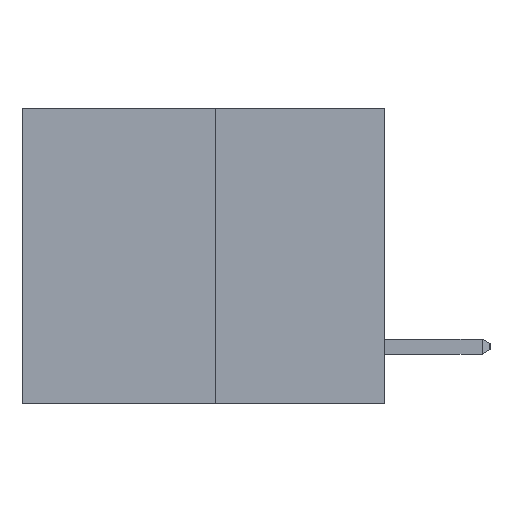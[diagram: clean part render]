
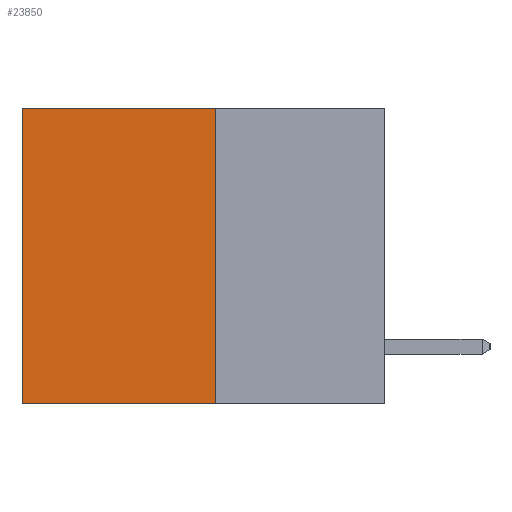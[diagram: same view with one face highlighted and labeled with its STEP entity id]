
A CAD part, left-side view. The second image highlights one B-rep face of the part: STEP entity #23850.
In plain terms, the highlighted planar face has unit normal (-1, 0, 0).
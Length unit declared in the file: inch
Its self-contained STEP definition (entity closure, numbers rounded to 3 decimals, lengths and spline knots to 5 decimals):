
#1382 = FACE_OUTER_BOUND ( 'NONE', #16601, .T. ) ;
#1690 = LINE ( 'NONE', #16212, #13987 ) ;
#6266 = CARTESIAN_POINT ( 'NONE',  ( 0.3165, 0.28, -0.49 ) ) ;
#6625 = VERTEX_POINT ( 'NONE', #8725 ) ;
#7348 = LINE ( 'NONE', #9568, #12808 ) ;
#7828 = PLANE ( 'NONE',  #15350 ) ;
#8725 = CARTESIAN_POINT ( 'NONE',  ( 0.3165, 0.28, 0. ) ) ;
#9127 = VERTEX_POINT ( 'NONE', #21963 ) ;
#9568 = CARTESIAN_POINT ( 'NONE',  ( 0.3165, 0.6, -0.49 ) ) ;
#9924 = DIRECTION ( 'NONE',  ( 0., 0., -1. ) ) ;
#10019 = CARTESIAN_POINT ( 'NONE',  ( 0.3165, 0.28, -0.49 ) ) ;
#11030 = EDGE_CURVE ( 'NONE', #23830, #9127, #7348, .T. ) ;
#11343 = DIRECTION ( 'NONE',  ( 0., 0., -1. ) ) ;
#11978 = DIRECTION ( 'NONE',  ( 0., 0., -1. ) ) ;
#12808 = VECTOR ( 'NONE', #11343, 39.37008 ) ;
#13666 = EDGE_CURVE ( 'NONE', #6625, #14629, #18424, .T. ) ;
#13949 = CARTESIAN_POINT ( 'NONE',  ( 0.3165, 0.28, -0.49 ) ) ;
#13987 = VECTOR ( 'NONE', #17715, 39.37008 ) ;
#14253 = LINE ( 'NONE', #16948, #17502 ) ;
#14288 = VECTOR ( 'NONE', #9924, 39.37008 ) ;
#14629 = VERTEX_POINT ( 'NONE', #6266 ) ;
#15350 = AXIS2_PLACEMENT_3D ( 'NONE', #10019, #17778, #11978 ) ;
#15754 = ORIENTED_EDGE ( 'NONE', *, *, #11030, .T. ) ;
#16212 = CARTESIAN_POINT ( 'NONE',  ( 0.3165, 0.28, -0.49 ) ) ;
#16601 = EDGE_LOOP ( 'NONE', ( #15754, #18863, #17419, #18493 ) ) ;
#16948 = CARTESIAN_POINT ( 'NONE',  ( 0.3165, 0.28, 0. ) ) ;
#17419 = ORIENTED_EDGE ( 'NONE', *, *, #13666, .F. ) ;
#17502 = VECTOR ( 'NONE', #18851, 39.37008 ) ;
#17593 = CARTESIAN_POINT ( 'NONE',  ( 0.3165, 0.6, 0. ) ) ;
#17715 = DIRECTION ( 'NONE',  ( 0., 1., 0. ) ) ;
#17778 = DIRECTION ( 'NONE',  ( 1., 0., 0. ) ) ;
#18424 = LINE ( 'NONE', #13949, #14288 ) ;
#18493 = ORIENTED_EDGE ( 'NONE', *, *, #24210, .T. ) ;
#18851 = DIRECTION ( 'NONE',  ( 0., 1., 0. ) ) ;
#18863 = ORIENTED_EDGE ( 'NONE', *, *, #23527, .F. ) ;
#21963 = CARTESIAN_POINT ( 'NONE',  ( 0.3165, 0.6, -0.49 ) ) ;
#23527 = EDGE_CURVE ( 'NONE', #14629, #9127, #1690, .T. ) ;
#23830 = VERTEX_POINT ( 'NONE', #17593 ) ;
#23850 = ADVANCED_FACE ( 'NONE', ( #1382 ), #7828, .F. ) ;
#24210 = EDGE_CURVE ( 'NONE', #6625, #23830, #14253, .T. ) ;
